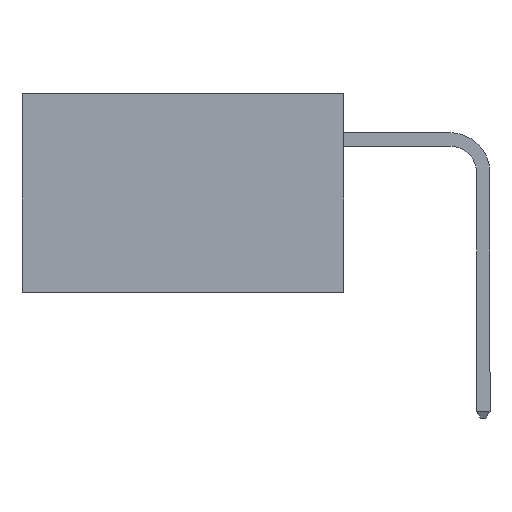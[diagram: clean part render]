
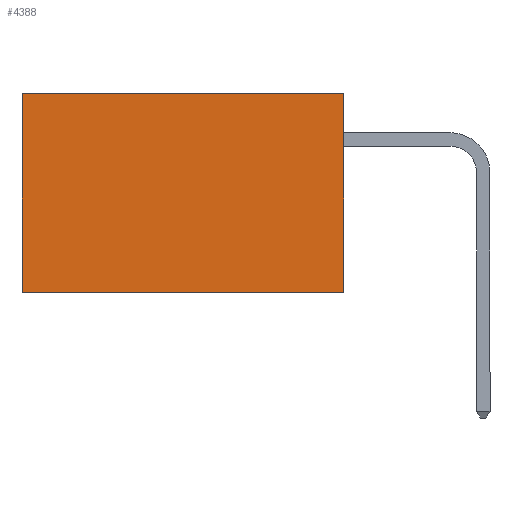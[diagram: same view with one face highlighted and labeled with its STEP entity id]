
A CAD part, left-side view. The second image highlights one B-rep face of the part: STEP entity #4388.
In plain terms, the highlighted planar face has unit normal (-1, 0, 0).
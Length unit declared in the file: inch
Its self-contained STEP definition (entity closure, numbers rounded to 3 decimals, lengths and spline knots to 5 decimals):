
#315 = DIRECTION ( 'NONE',  ( 0., 1., 0. ) ) ;
#596 = LINE ( 'NONE', #3421, #5550 ) ;
#695 = LINE ( 'NONE', #1386, #5063 ) ;
#919 = EDGE_CURVE ( 'NONE', #3480, #5735, #4993, .T. ) ;
#1013 = DIRECTION ( 'NONE',  ( 0., 0., -1. ) ) ;
#1386 = CARTESIAN_POINT ( 'NONE',  ( 0.2615, 0.6, -0.37 ) ) ;
#1519 = VERTEX_POINT ( 'NONE', #2110 ) ;
#1613 = VECTOR ( 'NONE', #3607, 39.37008 ) ;
#1837 = LINE ( 'NONE', #6657, #5426 ) ;
#2110 = CARTESIAN_POINT ( 'NONE',  ( 0.2615, 0.6, -0.37 ) ) ;
#2347 = CARTESIAN_POINT ( 'NONE',  ( 0.2615, 0., -0.37 ) ) ;
#2403 = EDGE_CURVE ( 'NONE', #3480, #5185, #596, .T. ) ;
#2611 = ORIENTED_EDGE ( 'NONE', *, *, #5159, .T. ) ;
#3421 = CARTESIAN_POINT ( 'NONE',  ( 0.2615, 0., -0.37 ) ) ;
#3480 = VERTEX_POINT ( 'NONE', #8017 ) ;
#3498 = DIRECTION ( 'NONE',  ( 0., 0., -1. ) ) ;
#3607 = DIRECTION ( 'NONE',  ( 0., 1., 0. ) ) ;
#3633 = ORIENTED_EDGE ( 'NONE', *, *, #2403, .F. ) ;
#3745 = PLANE ( 'NONE',  #7753 ) ;
#4044 = EDGE_CURVE ( 'NONE', #5185, #1519, #1837, .T. ) ;
#4388 = ADVANCED_FACE ( 'NONE', ( #6736 ), #3745, .F. ) ;
#4683 = DIRECTION ( 'NONE',  ( 0., 0., -1. ) ) ;
#4993 = LINE ( 'NONE', #5184, #1613 ) ;
#5063 = VECTOR ( 'NONE', #3498, 39.37008 ) ;
#5159 = EDGE_CURVE ( 'NONE', #5735, #1519, #695, .T. ) ;
#5184 = CARTESIAN_POINT ( 'NONE',  ( 0.2615, 0., 0. ) ) ;
#5185 = VERTEX_POINT ( 'NONE', #5745 ) ;
#5426 = VECTOR ( 'NONE', #315, 39.37008 ) ;
#5550 = VECTOR ( 'NONE', #4683, 39.37008 ) ;
#5735 = VERTEX_POINT ( 'NONE', #8919 ) ;
#5745 = CARTESIAN_POINT ( 'NONE',  ( 0.2615, 0., -0.37 ) ) ;
#6020 = ORIENTED_EDGE ( 'NONE', *, *, #4044, .F. ) ;
#6599 = DIRECTION ( 'NONE',  ( 1., 0., 0. ) ) ;
#6657 = CARTESIAN_POINT ( 'NONE',  ( 0.2615, 0., -0.37 ) ) ;
#6736 = FACE_OUTER_BOUND ( 'NONE', #7342, .T. ) ;
#7342 = EDGE_LOOP ( 'NONE', ( #2611, #6020, #3633, #7643 ) ) ;
#7643 = ORIENTED_EDGE ( 'NONE', *, *, #919, .T. ) ;
#7753 = AXIS2_PLACEMENT_3D ( 'NONE', #2347, #6599, #1013 ) ;
#8017 = CARTESIAN_POINT ( 'NONE',  ( 0.2615, 0., 0. ) ) ;
#8919 = CARTESIAN_POINT ( 'NONE',  ( 0.2615, 0.6, 0. ) ) ;
